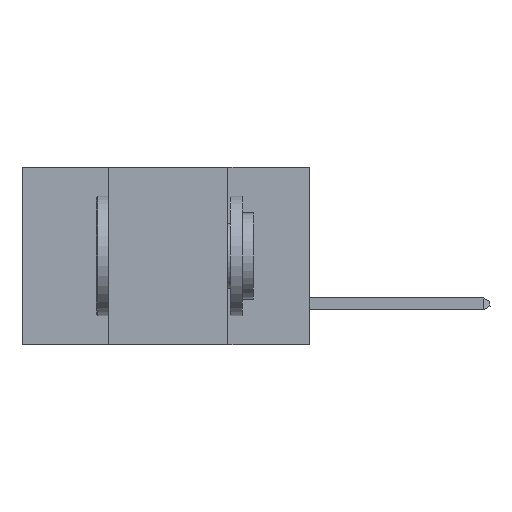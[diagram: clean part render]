
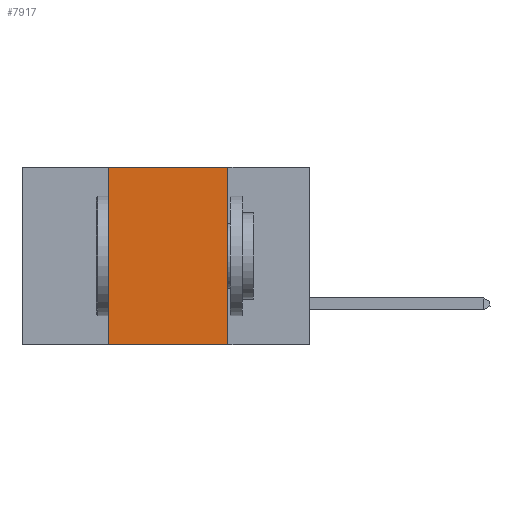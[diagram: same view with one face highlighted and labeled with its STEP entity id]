
A CAD part, left-side view. The second image highlights one B-rep face of the part: STEP entity #7917.
In plain terms, the highlighted planar face has unit normal (-1, 0, 0).
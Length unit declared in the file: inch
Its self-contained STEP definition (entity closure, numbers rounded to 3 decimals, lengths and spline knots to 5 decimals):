
#8 = DIRECTION ( 'NONE',  ( 0., -1., 0. ) ) ;
#131 = ORIENTED_EDGE ( 'NONE', *, *, #2541, .T. ) ;
#1130 = DIRECTION ( 'NONE',  ( 0., 0., -1. ) ) ;
#1173 = VECTOR ( 'NONE', #8, 39.37008 ) ;
#1621 = VECTOR ( 'NONE', #3156, 39.37008 ) ;
#1803 = CARTESIAN_POINT ( 'NONE',  ( 0., 0.17, 0. ) ) ;
#1881 = CARTESIAN_POINT ( 'NONE',  ( 0., 0.6, -0.37 ) ) ;
#2541 = EDGE_CURVE ( 'NONE', #11030, #2580, #11979, .T. ) ;
#2580 = VERTEX_POINT ( 'NONE', #11212 ) ;
#2794 = ORIENTED_EDGE ( 'NONE', *, *, #5385, .F. ) ;
#2839 = DIRECTION ( 'NONE',  ( 0., -1., 0. ) ) ;
#3148 = AXIS2_PLACEMENT_3D ( 'NONE', #5889, #3902, #1130 ) ;
#3156 = DIRECTION ( 'NONE',  ( 0., 0., 1. ) ) ;
#3663 = LINE ( 'NONE', #5627, #1173 ) ;
#3902 = DIRECTION ( 'NONE',  ( 1., 0., 0. ) ) ;
#4097 = LINE ( 'NONE', #10550, #1621 ) ;
#4572 = VECTOR ( 'NONE', #2839, 39.37008 ) ;
#5063 = FACE_OUTER_BOUND ( 'NONE', #5880, .T. ) ;
#5112 = ORIENTED_EDGE ( 'NONE', *, *, #7949, .F. ) ;
#5385 = EDGE_CURVE ( 'NONE', #7640, #7396, #3663, .T. ) ;
#5627 = CARTESIAN_POINT ( 'NONE',  ( 0., 0.6, 0. ) ) ;
#5880 = EDGE_LOOP ( 'NONE', ( #5112, #2794, #11673, #131 ) ) ;
#5889 = CARTESIAN_POINT ( 'NONE',  ( 0., 0.6, 0. ) ) ;
#6247 = CARTESIAN_POINT ( 'NONE',  ( 0., 0.42, 0. ) ) ;
#6263 = EDGE_CURVE ( 'NONE', #11030, #7640, #4097, .T. ) ;
#6687 = VECTOR ( 'NONE', #10861, 39.37008 ) ;
#7396 = VERTEX_POINT ( 'NONE', #1803 ) ;
#7640 = VERTEX_POINT ( 'NONE', #6247 ) ;
#7775 = CARTESIAN_POINT ( 'NONE',  ( 0., 0.42, -0.37 ) ) ;
#7917 = ADVANCED_FACE ( 'NONE', ( #5063 ), #10251, .F. ) ;
#7949 = EDGE_CURVE ( 'NONE', #7396, #2580, #8997, .T. ) ;
#8146 = CARTESIAN_POINT ( 'NONE',  ( 0., 0.17, 0. ) ) ;
#8997 = LINE ( 'NONE', #8146, #6687 ) ;
#10251 = PLANE ( 'NONE',  #3148 ) ;
#10550 = CARTESIAN_POINT ( 'NONE',  ( 0., 0.42, 0. ) ) ;
#10861 = DIRECTION ( 'NONE',  ( 0., 0., -1. ) ) ;
#11030 = VERTEX_POINT ( 'NONE', #7775 ) ;
#11212 = CARTESIAN_POINT ( 'NONE',  ( 0., 0.17, -0.37 ) ) ;
#11673 = ORIENTED_EDGE ( 'NONE', *, *, #6263, .F. ) ;
#11979 = LINE ( 'NONE', #1881, #4572 ) ;
